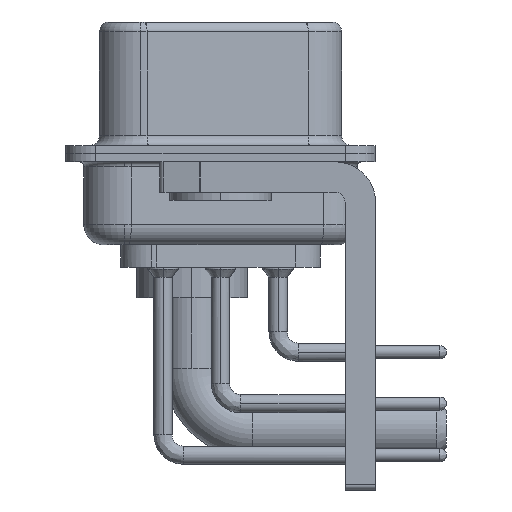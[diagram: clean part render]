
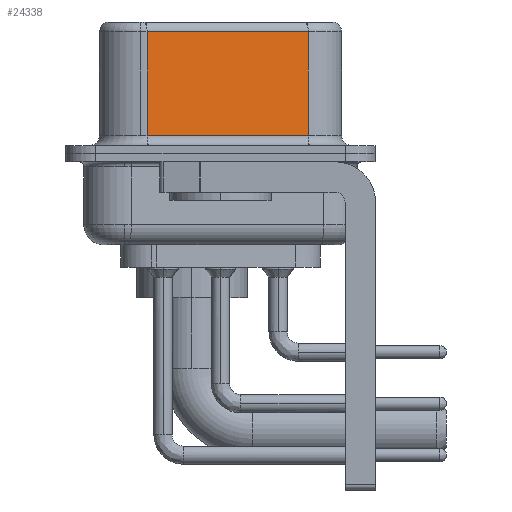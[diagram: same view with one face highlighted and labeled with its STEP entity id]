
A CAD part, left-side view. The second image highlights one B-rep face of the part: STEP entity #24338.
In plain terms, the highlighted planar face has unit normal (-0.985, -0.174, 0).
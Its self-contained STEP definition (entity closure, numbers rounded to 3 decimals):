
#20 = VERTEX_POINT ( 'NONE', #2274 ) ;
#255 = ORIENTED_EDGE ( 'NONE', *, *, #32092, .F. ) ;
#2274 = CARTESIAN_POINT ( 'NONE',  ( 3.73, 3.628, 0.9 ) ) ;
#5619 = VERTEX_POINT ( 'NONE', #21612 ) ;
#6726 = DIRECTION ( 'NONE',  ( -0.174, 0.985, 0. ) ) ;
#7043 = CARTESIAN_POINT ( 'NONE',  ( 5.132, -4.322, 6.52 ) ) ;
#7395 = CARTESIAN_POINT ( 'NONE',  ( 5.132, -4.322, 0.9 ) ) ;
#8092 = ORIENTED_EDGE ( 'NONE', *, *, #23012, .T. ) ;
#9207 = EDGE_LOOP ( 'NONE', ( #255, #20095, #25472, #8092 ) ) ;
#10214 = LINE ( 'NONE', #7395, #25711 ) ;
#10217 = DIRECTION ( 'NONE',  ( -0.174, 0.985, 0. ) ) ;
#10525 = VECTOR ( 'NONE', #11322, 1000. ) ;
#10569 = FACE_OUTER_BOUND ( 'NONE', #9207, .T. ) ;
#11322 = DIRECTION ( 'NONE',  ( 0., 0., -1. ) ) ;
#13065 = CARTESIAN_POINT ( 'NONE',  ( 5.132, -4.322, 6.02 ) ) ;
#14133 = LINE ( 'NONE', #25543, #10525 ) ;
#14682 = EDGE_CURVE ( 'NONE', #36954, #33089, #20920, .T. ) ;
#18308 = EDGE_CURVE ( 'NONE', #33089, #20, #14133, .T. ) ;
#18823 = DIRECTION ( 'NONE',  ( 0.985, 0.174, 0. ) ) ;
#20095 = ORIENTED_EDGE ( 'NONE', *, *, #14682, .T. ) ;
#20920 = LINE ( 'NONE', #32366, #21092 ) ;
#21092 = VECTOR ( 'NONE', #6726, 1000. ) ;
#21239 = DIRECTION ( 'NONE',  ( 0., 0., -1. ) ) ;
#21612 = CARTESIAN_POINT ( 'NONE',  ( 5.132, -4.322, 0.9 ) ) ;
#23012 = EDGE_CURVE ( 'NONE', #20, #5619, #10214, .T. ) ;
#24239 = PLANE ( 'NONE',  #25795 ) ;
#24338 = ADVANCED_FACE ( 'NONE', ( #10569 ), #24239, .F. ) ;
#25472 = ORIENTED_EDGE ( 'NONE', *, *, #18308, .T. ) ;
#25543 = CARTESIAN_POINT ( 'NONE',  ( 3.73, 3.628, 6.52 ) ) ;
#25711 = VECTOR ( 'NONE', #36026, 1000. ) ;
#25795 = AXIS2_PLACEMENT_3D ( 'NONE', #7043, #18823, #10217 ) ;
#26856 = LINE ( 'NONE', #30045, #31560 ) ;
#30045 = CARTESIAN_POINT ( 'NONE',  ( 5.132, -4.322, 6.52 ) ) ;
#31560 = VECTOR ( 'NONE', #21239, 1000. ) ;
#32092 = EDGE_CURVE ( 'NONE', #36954, #5619, #26856, .T. ) ;
#32366 = CARTESIAN_POINT ( 'NONE',  ( 5.132, -4.322, 6.02 ) ) ;
#33089 = VERTEX_POINT ( 'NONE', #33306 ) ;
#33306 = CARTESIAN_POINT ( 'NONE',  ( 3.73, 3.628, 6.02 ) ) ;
#36026 = DIRECTION ( 'NONE',  ( 0.174, -0.985, 0. ) ) ;
#36954 = VERTEX_POINT ( 'NONE', #13065 ) ;
